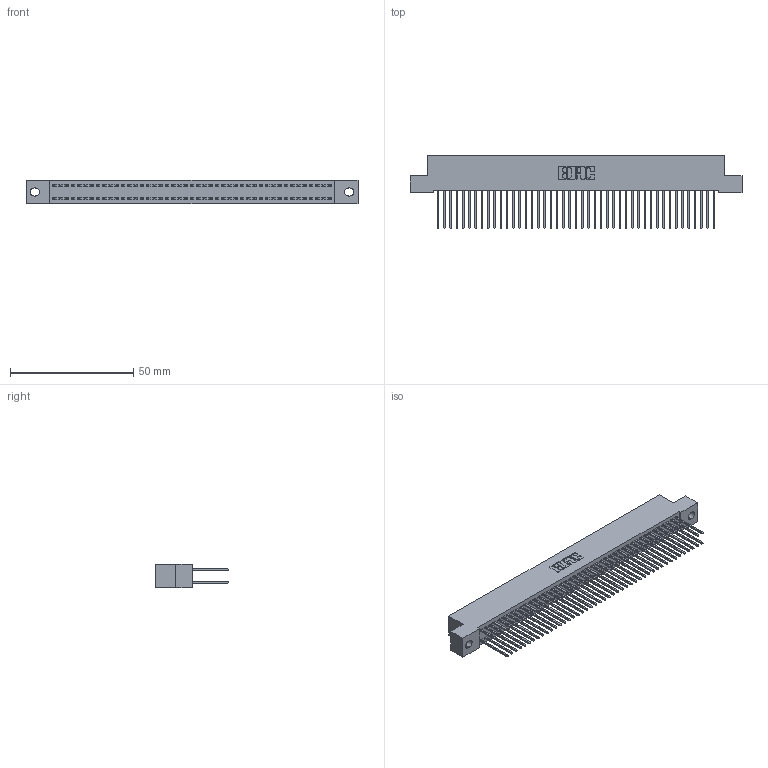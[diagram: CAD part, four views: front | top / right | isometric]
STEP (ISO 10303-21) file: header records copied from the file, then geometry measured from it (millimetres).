
FILE_DESCRIPTION (( 'STEP AP203' ), '1' );
FILE_NAME ('342-090-540-202.STEP', '2018-08-14T01:04:46', ( '' ), ( '' ), 'SwSTEP 2.0', 'SolidWorks 2016', '' );
FILE_SCHEMA (( 'CONFIG_CONTROL_DESIGN' ));
Length unit declared in the file: inch
Products named in the file (3): 342-090-540-202; 342 Part_.128 Slot; 345-292-001_345-293-140
Assembly tree (91 placements, depth 2):
  342-090-540-202
    342 Part_.128 Slot
    345-292-001_345-293-140  x90
Bounding box: 134.62 x 29.47 x 9.4 mm (x, y, z)
Volume: 12398.8 mm3; surface area: 21532.4 mm2
Topology: 91 solids, 91 shells, 4794 faces, 14261 edges, 9386 vertices
Faces by surface type: plane 3310, cylinder 1484
Entity records: 28583 total; most frequent: CARTESIAN_POINT 4734, ORIENTED_EDGE 4670, DIRECTION 4039, EDGE_CURVE 2335, VECTOR 2207, LINE 2207, VERTEX_POINT 1554, AXIS2_PLACEMENT_3D 916
